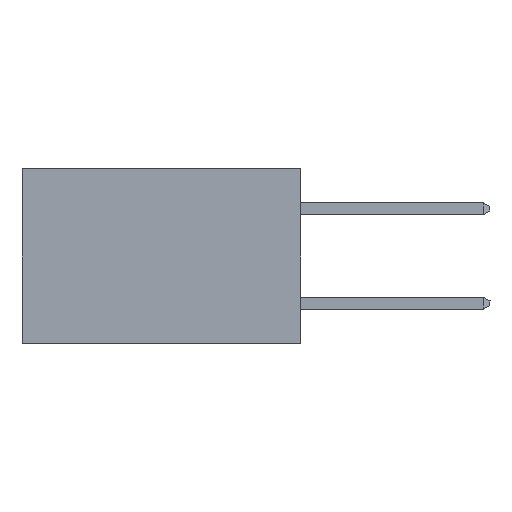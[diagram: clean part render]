
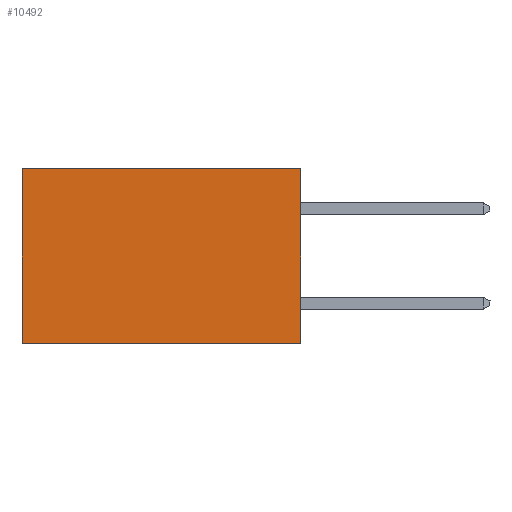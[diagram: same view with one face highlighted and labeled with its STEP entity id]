
A CAD part, left-side view. The second image highlights one B-rep face of the part: STEP entity #10492.
In plain terms, the highlighted planar face has unit normal (-1, 0, 0).
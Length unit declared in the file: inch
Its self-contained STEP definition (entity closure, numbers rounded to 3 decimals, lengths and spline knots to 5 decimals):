
#328 = CARTESIAN_POINT ( 'NONE',  ( 0.277, 0., -0.37 ) ) ;
#353 = VECTOR ( 'NONE', #10920, 39.37008 ) ;
#627 = CARTESIAN_POINT ( 'NONE',  ( 0.277, 0., 0. ) ) ;
#776 = ORIENTED_EDGE ( 'NONE', *, *, #2597, .T. ) ;
#1759 = EDGE_CURVE ( 'NONE', #27576, #14836, #7078, .T. ) ;
#2511 = DIRECTION ( 'NONE',  ( 1., 0., 0. ) ) ;
#2546 = CARTESIAN_POINT ( 'NONE',  ( 0.277, 0., -0.37 ) ) ;
#2597 = EDGE_CURVE ( 'NONE', #6004, #27576, #12557, .T. ) ;
#3087 = CARTESIAN_POINT ( 'NONE',  ( 0.277, 0.59, 0. ) ) ;
#3796 = VECTOR ( 'NONE', #16577, 39.37008 ) ;
#4462 = LINE ( 'NONE', #7944, #3796 ) ;
#5536 = LINE ( 'NONE', #20576, #17717 ) ;
#6004 = VERTEX_POINT ( 'NONE', #20452 ) ;
#7078 = LINE ( 'NONE', #15448, #23559 ) ;
#7653 = DIRECTION ( 'NONE',  ( 0., 1., 0. ) ) ;
#7944 = CARTESIAN_POINT ( 'NONE',  ( 0.277, 0., -0.37 ) ) ;
#10492 = ADVANCED_FACE ( 'NONE', ( #23146 ), #26013, .F. ) ;
#10920 = DIRECTION ( 'NONE',  ( 0., 1., 0. ) ) ;
#11557 = CARTESIAN_POINT ( 'NONE',  ( 0.277, 0.59, -0.37 ) ) ;
#12468 = EDGE_CURVE ( 'NONE', #17903, #14836, #5536, .T. ) ;
#12557 = LINE ( 'NONE', #627, #353 ) ;
#14354 = EDGE_CURVE ( 'NONE', #6004, #17903, #4462, .T. ) ;
#14836 = VERTEX_POINT ( 'NONE', #11557 ) ;
#15219 = DIRECTION ( 'NONE',  ( 0., 0., -1. ) ) ;
#15448 = CARTESIAN_POINT ( 'NONE',  ( 0.277, 0.59, -0.37 ) ) ;
#16577 = DIRECTION ( 'NONE',  ( 0., 0., -1. ) ) ;
#17606 = DIRECTION ( 'NONE',  ( 0., 0., -1. ) ) ;
#17717 = VECTOR ( 'NONE', #7653, 39.37008 ) ;
#17903 = VERTEX_POINT ( 'NONE', #2546 ) ;
#17920 = ORIENTED_EDGE ( 'NONE', *, *, #1759, .T. ) ;
#18543 = ORIENTED_EDGE ( 'NONE', *, *, #12468, .F. ) ;
#19071 = ORIENTED_EDGE ( 'NONE', *, *, #14354, .F. ) ;
#20452 = CARTESIAN_POINT ( 'NONE',  ( 0.277, 0., 0. ) ) ;
#20576 = CARTESIAN_POINT ( 'NONE',  ( 0.277, 0., -0.37 ) ) ;
#22642 = AXIS2_PLACEMENT_3D ( 'NONE', #328, #2511, #17606 ) ;
#23146 = FACE_OUTER_BOUND ( 'NONE', #27624, .T. ) ;
#23559 = VECTOR ( 'NONE', #15219, 39.37008 ) ;
#26013 = PLANE ( 'NONE',  #22642 ) ;
#27576 = VERTEX_POINT ( 'NONE', #3087 ) ;
#27624 = EDGE_LOOP ( 'NONE', ( #17920, #18543, #19071, #776 ) ) ;
